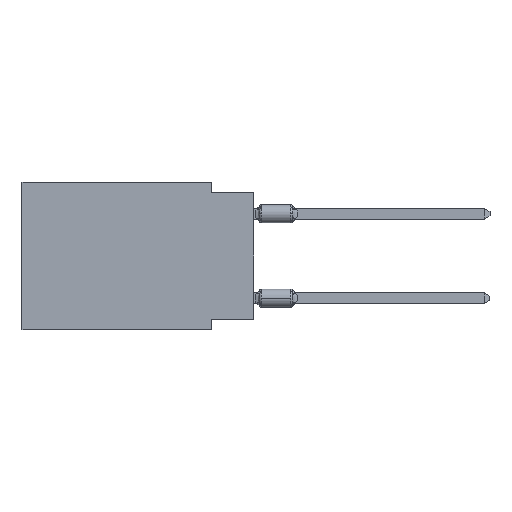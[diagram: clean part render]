
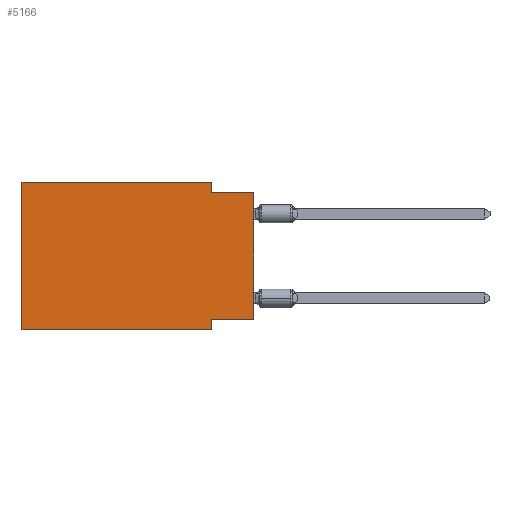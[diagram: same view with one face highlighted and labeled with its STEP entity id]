
A CAD part, left-side view. The second image highlights one B-rep face of the part: STEP entity #5166.
In plain terms, the highlighted planar face has unit normal (-1, 0, 0).
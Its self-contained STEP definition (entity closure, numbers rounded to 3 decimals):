
#778 = CARTESIAN_POINT ( 'NONE',  ( 0., 0., -8.255 ) ) ;
#857 = CARTESIAN_POINT ( 'NONE',  ( 0., 2.54, -8.89 ) ) ;
#904 = ORIENTED_EDGE ( 'NONE', *, *, #6329, .F. ) ;
#1194 = LINE ( 'NONE', #13500, #20041 ) ;
#1924 = CARTESIAN_POINT ( 'NONE',  ( 0., 13.97, 0. ) ) ;
#2162 = CARTESIAN_POINT ( 'NONE',  ( 0., 2.54, -8.89 ) ) ;
#2858 = CARTESIAN_POINT ( 'NONE',  ( 0., 13.97, 0. ) ) ;
#3038 = VERTEX_POINT ( 'NONE', #5882 ) ;
#3303 = ORIENTED_EDGE ( 'NONE', *, *, #13056, .F. ) ;
#3311 = EDGE_CURVE ( 'NONE', #21102, #19833, #10761, .T. ) ;
#3878 = DIRECTION ( 'NONE',  ( 0., -1., 0. ) ) ;
#4100 = VECTOR ( 'NONE', #14867, 1000. ) ;
#4428 = ORIENTED_EDGE ( 'NONE', *, *, #6180, .F. ) ;
#4620 = VECTOR ( 'NONE', #3878, 1000. ) ;
#5166 = ADVANCED_FACE ( 'NONE', ( #14459 ), #21488, .F. ) ;
#5710 = DIRECTION ( 'NONE',  ( 1., 0., 0. ) ) ;
#5768 = VERTEX_POINT ( 'NONE', #15999 ) ;
#5882 = CARTESIAN_POINT ( 'NONE',  ( 0., 2.54, -8.255 ) ) ;
#6180 = EDGE_CURVE ( 'NONE', #21102, #8016, #18089, .T. ) ;
#6329 = EDGE_CURVE ( 'NONE', #5768, #20174, #12283, .T. ) ;
#6640 = AXIS2_PLACEMENT_3D ( 'NONE', #1924, #5710, #12724 ) ;
#6682 = VERTEX_POINT ( 'NONE', #13328 ) ;
#6701 = CARTESIAN_POINT ( 'NONE',  ( 0., 0., -8.255 ) ) ;
#7140 = EDGE_LOOP ( 'NONE', ( #21158, #11858, #904, #19357, #4428, #20606, #9216, #3303 ) ) ;
#7235 = DIRECTION ( 'NONE',  ( 0., 0., -1. ) ) ;
#7676 = LINE ( 'NONE', #2162, #19618 ) ;
#8016 = VERTEX_POINT ( 'NONE', #9044 ) ;
#8149 = VECTOR ( 'NONE', #7235, 1000. ) ;
#8194 = DIRECTION ( 'NONE',  ( 0., 0., 1. ) ) ;
#8951 = CARTESIAN_POINT ( 'NONE',  ( 0., 2.54, 0. ) ) ;
#9044 = CARTESIAN_POINT ( 'NONE',  ( 0., 13.97, 0. ) ) ;
#9216 = ORIENTED_EDGE ( 'NONE', *, *, #10099, .F. ) ;
#9822 = VECTOR ( 'NONE', #19025, 1000. ) ;
#10099 = EDGE_CURVE ( 'NONE', #3038, #19833, #7676, .T. ) ;
#10586 = EDGE_CURVE ( 'NONE', #21156, #6682, #1194, .T. ) ;
#10761 = LINE ( 'NONE', #17925, #12076 ) ;
#11100 = EDGE_CURVE ( 'NONE', #20174, #6682, #17941, .T. ) ;
#11858 = ORIENTED_EDGE ( 'NONE', *, *, #11100, .F. ) ;
#11985 = LINE ( 'NONE', #6701, #9822 ) ;
#12076 = VECTOR ( 'NONE', #20211, 1000. ) ;
#12283 = LINE ( 'NONE', #8951, #8149 ) ;
#12724 = DIRECTION ( 'NONE',  ( 0., 0., -1. ) ) ;
#13056 = EDGE_CURVE ( 'NONE', #21156, #3038, #11985, .T. ) ;
#13328 = CARTESIAN_POINT ( 'NONE',  ( 0., 0., -0.635 ) ) ;
#13500 = CARTESIAN_POINT ( 'NONE',  ( 0., 0., 0. ) ) ;
#14013 = CARTESIAN_POINT ( 'NONE',  ( 0., 0., -0.635 ) ) ;
#14459 = FACE_OUTER_BOUND ( 'NONE', #7140, .T. ) ;
#14644 = VECTOR ( 'NONE', #18837, 1000. ) ;
#14706 = DIRECTION ( 'NONE',  ( 0., 0., -1. ) ) ;
#14867 = DIRECTION ( 'NONE',  ( 0., 0., 1. ) ) ;
#15234 = EDGE_CURVE ( 'NONE', #8016, #5768, #19067, .T. ) ;
#15960 = CARTESIAN_POINT ( 'NONE',  ( 0., 13.97, -8.89 ) ) ;
#15999 = CARTESIAN_POINT ( 'NONE',  ( 0., 2.54, 0. ) ) ;
#17925 = CARTESIAN_POINT ( 'NONE',  ( 0., 13.97, -8.89 ) ) ;
#17941 = LINE ( 'NONE', #14013, #4620 ) ;
#18089 = LINE ( 'NONE', #19691, #4100 ) ;
#18837 = DIRECTION ( 'NONE',  ( 0., -1., 0. ) ) ;
#19025 = DIRECTION ( 'NONE',  ( 0., 1., 0. ) ) ;
#19067 = LINE ( 'NONE', #2858, #14644 ) ;
#19357 = ORIENTED_EDGE ( 'NONE', *, *, #15234, .F. ) ;
#19618 = VECTOR ( 'NONE', #14706, 1000. ) ;
#19691 = CARTESIAN_POINT ( 'NONE',  ( 0., 13.97, 0. ) ) ;
#19833 = VERTEX_POINT ( 'NONE', #857 ) ;
#20041 = VECTOR ( 'NONE', #8194, 1000. ) ;
#20174 = VERTEX_POINT ( 'NONE', #22683 ) ;
#20211 = DIRECTION ( 'NONE',  ( 0., -1., 0. ) ) ;
#20606 = ORIENTED_EDGE ( 'NONE', *, *, #3311, .T. ) ;
#21102 = VERTEX_POINT ( 'NONE', #15960 ) ;
#21156 = VERTEX_POINT ( 'NONE', #778 ) ;
#21158 = ORIENTED_EDGE ( 'NONE', *, *, #10586, .T. ) ;
#21488 = PLANE ( 'NONE',  #6640 ) ;
#22683 = CARTESIAN_POINT ( 'NONE',  ( 0., 2.54, -0.635 ) ) ;
